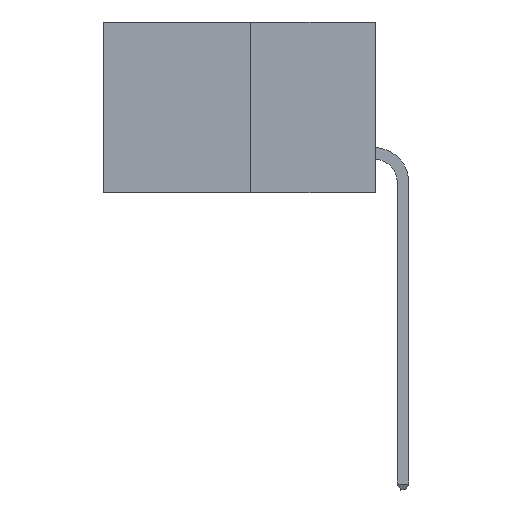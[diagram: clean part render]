
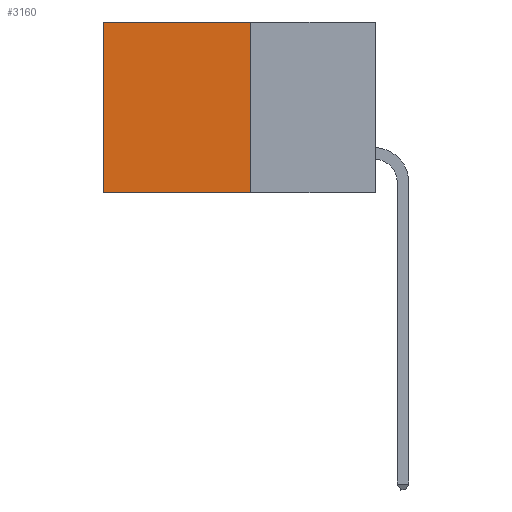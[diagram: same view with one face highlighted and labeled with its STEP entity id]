
A CAD part, left-side view. The second image highlights one B-rep face of the part: STEP entity #3160.
In plain terms, the highlighted planar face has unit normal (-1, 0, 0).
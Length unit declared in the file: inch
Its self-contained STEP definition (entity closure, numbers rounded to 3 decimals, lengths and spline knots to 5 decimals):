
#64 = DIRECTION ( 'NONE',  ( 0., 1., 0. ) ) ;
#698 = CARTESIAN_POINT ( 'NONE',  ( 0.277, 0.59, 0. ) ) ;
#2771 = DIRECTION ( 'NONE',  ( 0., 0., -1. ) ) ;
#3160 = ADVANCED_FACE ( 'NONE', ( #21373 ), #3994, .F. ) ;
#3200 = VECTOR ( 'NONE', #2771, 39.37008 ) ;
#3203 = VECTOR ( 'NONE', #14637, 39.37008 ) ;
#3333 = ORIENTED_EDGE ( 'NONE', *, *, #22867, .F. ) ;
#3364 = CARTESIAN_POINT ( 'NONE',  ( 0.277, 0.27, -0.37 ) ) ;
#3395 = ORIENTED_EDGE ( 'NONE', *, *, #22128, .F. ) ;
#3812 = DIRECTION ( 'NONE',  ( 0., 0., -1. ) ) ;
#3881 = DIRECTION ( 'NONE',  ( 1., 0., 0. ) ) ;
#3994 = PLANE ( 'NONE',  #25778 ) ;
#4111 = CARTESIAN_POINT ( 'NONE',  ( 0.277, 0.27, -0.37 ) ) ;
#6166 = EDGE_CURVE ( 'NONE', #17913, #7976, #18670, .T. ) ;
#7221 = VECTOR ( 'NONE', #64, 39.37008 ) ;
#7387 = EDGE_LOOP ( 'NONE', ( #12920, #3395, #3333, #17452 ) ) ;
#7976 = VERTEX_POINT ( 'NONE', #698 ) ;
#8536 = CARTESIAN_POINT ( 'NONE',  ( 0.277, 0.27, 0. ) ) ;
#10313 = CARTESIAN_POINT ( 'NONE',  ( 0.277, 0.59, -0.37 ) ) ;
#12920 = ORIENTED_EDGE ( 'NONE', *, *, #14487, .T. ) ;
#13377 = CARTESIAN_POINT ( 'NONE',  ( 0.277, 0.27, -0.37 ) ) ;
#14487 = EDGE_CURVE ( 'NONE', #7976, #20212, #19614, .T. ) ;
#14521 = LINE ( 'NONE', #13377, #3200 ) ;
#14637 = DIRECTION ( 'NONE',  ( 0., 0., -1. ) ) ;
#14715 = DIRECTION ( 'NONE',  ( 0., 1., 0. ) ) ;
#17251 = VECTOR ( 'NONE', #14715, 39.37008 ) ;
#17452 = ORIENTED_EDGE ( 'NONE', *, *, #6166, .T. ) ;
#17913 = VERTEX_POINT ( 'NONE', #26816 ) ;
#17920 = LINE ( 'NONE', #25669, #17251 ) ;
#18670 = LINE ( 'NONE', #8536, #7221 ) ;
#19614 = LINE ( 'NONE', #10313, #3203 ) ;
#20212 = VERTEX_POINT ( 'NONE', #23069 ) ;
#21373 = FACE_OUTER_BOUND ( 'NONE', #7387, .T. ) ;
#22128 = EDGE_CURVE ( 'NONE', #25174, #20212, #17920, .T. ) ;
#22867 = EDGE_CURVE ( 'NONE', #17913, #25174, #14521, .T. ) ;
#23069 = CARTESIAN_POINT ( 'NONE',  ( 0.277, 0.59, -0.37 ) ) ;
#25174 = VERTEX_POINT ( 'NONE', #3364 ) ;
#25669 = CARTESIAN_POINT ( 'NONE',  ( 0.277, 0.27, -0.37 ) ) ;
#25778 = AXIS2_PLACEMENT_3D ( 'NONE', #4111, #3881, #3812 ) ;
#26816 = CARTESIAN_POINT ( 'NONE',  ( 0.277, 0.27, 0. ) ) ;
